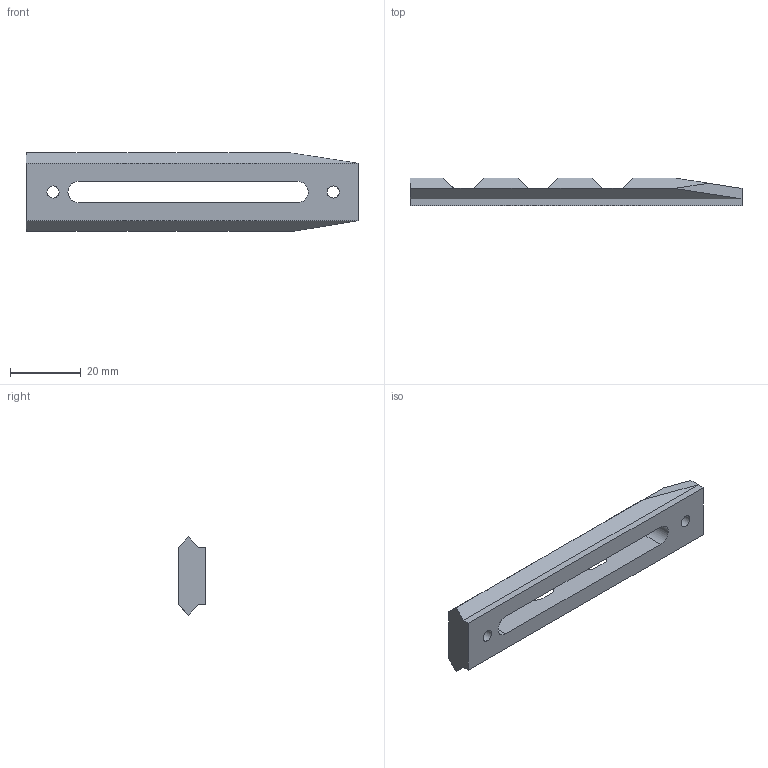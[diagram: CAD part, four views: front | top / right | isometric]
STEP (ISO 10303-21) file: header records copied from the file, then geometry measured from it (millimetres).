
FILE_DESCRIPTION (( 'STEP AP203' ), '1' );
FILE_NAME ('top_rail.STEP', '2020-05-10T05:53:28', ( '' ), ( '' ), 'SwSTEP 2.0', 'SolidWorks 2016', '' );
FILE_SCHEMA (( 'CONFIG_CONTROL_DESIGN' ));
Length unit declared in the file: millimetre
Products named in the file (1): top_rail
Bounding box: 93.62 x 7.86 x 22.05 mm (x, y, z)
Volume: 8575 mm3; surface area: 5449 mm2
Topology: 1 solids, 1 shells, 52 faces, 148 edges, 98 vertices
Faces by surface type: plane 46, cylinder 6
Full cylindrical faces by diameter (mm): 3.4 x2, 6.5 x2
Entity records: 1730 total; most frequent: CARTESIAN_POINT 308, ORIENTED_EDGE 286, DIRECTION 256, EDGE_CURVE 143, LINE 128, VECTOR 128, VERTEX_POINT 97, AXIS2_PLACEMENT_3D 64
